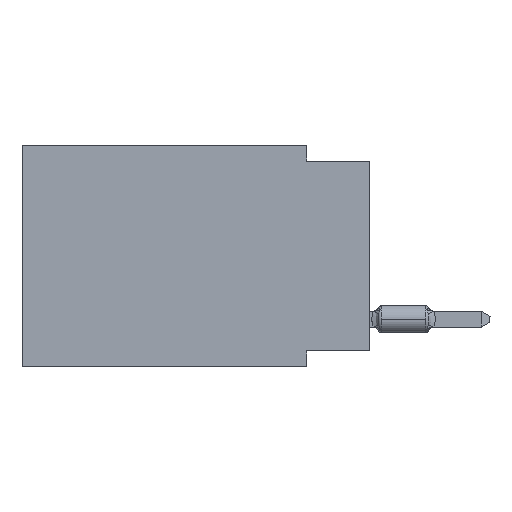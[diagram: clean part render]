
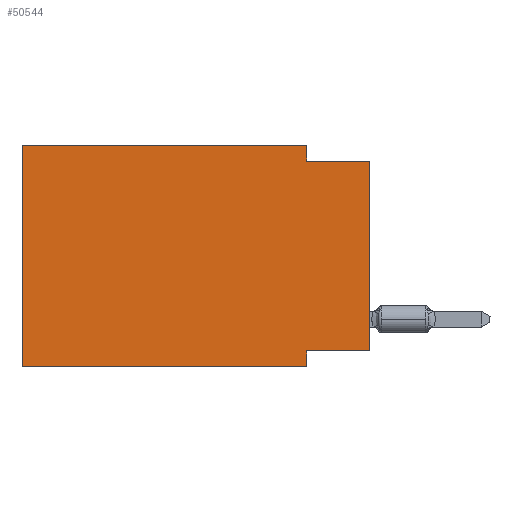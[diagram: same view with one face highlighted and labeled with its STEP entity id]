
A CAD part, left-side view. The second image highlights one B-rep face of the part: STEP entity #50544.
In plain terms, the highlighted planar face has unit normal (-1, 0, 0).
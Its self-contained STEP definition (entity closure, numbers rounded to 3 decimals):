
#319 = VECTOR ( 'NONE', #43218, 1000. ) ;
#4841 = EDGE_CURVE ( 'NONE', #57369, #77281, #84560, .T. ) ;
#5226 = EDGE_CURVE ( 'NONE', #74141, #13665, #69751, .T. ) ;
#5270 = CARTESIAN_POINT ( 'NONE',  ( 0., 0., -8.255 ) ) ;
#10536 = LINE ( 'NONE', #33897, #319 ) ;
#12109 = LINE ( 'NONE', #74909, #73997 ) ;
#13665 = VERTEX_POINT ( 'NONE', #39696 ) ;
#14472 = CARTESIAN_POINT ( 'NONE',  ( 0., 13.97, 0. ) ) ;
#18237 = DIRECTION ( 'NONE',  ( 0., -1., 0. ) ) ;
#18654 = EDGE_CURVE ( 'NONE', #75126, #88670, #10536, .T. ) ;
#21568 = EDGE_LOOP ( 'NONE', ( #23411, #101276, #94183, #102520, #75475, #31586, #55959, #97567 ) ) ;
#23411 = ORIENTED_EDGE ( 'NONE', *, *, #63049, .T. ) ;
#25244 = PLANE ( 'NONE',  #90442 ) ;
#25369 = VECTOR ( 'NONE', #18237, 1000. ) ;
#26015 = VECTOR ( 'NONE', #51516, 1000. ) ;
#31586 = ORIENTED_EDGE ( 'NONE', *, *, #64441, .T. ) ;
#33897 = CARTESIAN_POINT ( 'NONE',  ( 0., 2.54, -8.89 ) ) ;
#34335 = LINE ( 'NONE', #57688, #25369 ) ;
#34514 = DIRECTION ( 'NONE',  ( 0., 1., 0. ) ) ;
#36077 = CARTESIAN_POINT ( 'NONE',  ( 0., 2.54, -8.89 ) ) ;
#37963 = VERTEX_POINT ( 'NONE', #46831 ) ;
#39696 = CARTESIAN_POINT ( 'NONE',  ( 0., 0., -0.635 ) ) ;
#40943 = CARTESIAN_POINT ( 'NONE',  ( 0., 2.54, 0. ) ) ;
#43218 = DIRECTION ( 'NONE',  ( 0., 0., -1. ) ) ;
#43226 = CARTESIAN_POINT ( 'NONE',  ( 0., 0., 0. ) ) ;
#46831 = CARTESIAN_POINT ( 'NONE',  ( 0., 0., -8.255 ) ) ;
#47972 = EDGE_CURVE ( 'NONE', #77281, #57215, #34335, .T. ) ;
#50544 = ADVANCED_FACE ( 'NONE', ( #65697 ), #25244, .F. ) ;
#51516 = DIRECTION ( 'NONE',  ( 0., 0., 1. ) ) ;
#55959 = ORIENTED_EDGE ( 'NONE', *, *, #18654, .F. ) ;
#57215 = VERTEX_POINT ( 'NONE', #78774 ) ;
#57369 = VERTEX_POINT ( 'NONE', #77749 ) ;
#57688 = CARTESIAN_POINT ( 'NONE',  ( 0., 13.97, 0. ) ) ;
#57933 = DIRECTION ( 'NONE',  ( 0., 0., -1. ) ) ;
#63049 = EDGE_CURVE ( 'NONE', #37963, #13665, #67582, .T. ) ;
#64441 = EDGE_CURVE ( 'NONE', #57369, #88670, #12109, .T. ) ;
#64946 = VECTOR ( 'NONE', #34514, 1000. ) ;
#65697 = FACE_OUTER_BOUND ( 'NONE', #21568, .T. ) ;
#66331 = LINE ( 'NONE', #40943, #99849 ) ;
#66732 = CARTESIAN_POINT ( 'NONE',  ( 0., 13.97, 0. ) ) ;
#67582 = LINE ( 'NONE', #43226, #26015 ) ;
#69309 = CARTESIAN_POINT ( 'NONE',  ( 0., 13.97, 0. ) ) ;
#69751 = LINE ( 'NONE', #78060, #100337 ) ;
#73997 = VECTOR ( 'NONE', #82205, 1000. ) ;
#74141 = VERTEX_POINT ( 'NONE', #76071 ) ;
#74909 = CARTESIAN_POINT ( 'NONE',  ( 0., 13.97, -8.89 ) ) ;
#75126 = VERTEX_POINT ( 'NONE', #96522 ) ;
#75475 = ORIENTED_EDGE ( 'NONE', *, *, #4841, .F. ) ;
#76071 = CARTESIAN_POINT ( 'NONE',  ( 0., 2.54, -0.635 ) ) ;
#77281 = VERTEX_POINT ( 'NONE', #69309 ) ;
#77749 = CARTESIAN_POINT ( 'NONE',  ( 0., 13.97, -8.89 ) ) ;
#77886 = LINE ( 'NONE', #5270, #64946 ) ;
#78060 = CARTESIAN_POINT ( 'NONE',  ( 0., 0., -0.635 ) ) ;
#78774 = CARTESIAN_POINT ( 'NONE',  ( 0., 2.54, 0. ) ) ;
#78849 = VECTOR ( 'NONE', #92340, 1000. ) ;
#82205 = DIRECTION ( 'NONE',  ( 0., -1., 0. ) ) ;
#84560 = LINE ( 'NONE', #14472, #78849 ) ;
#88189 = DIRECTION ( 'NONE',  ( 0., 0., -1. ) ) ;
#88670 = VERTEX_POINT ( 'NONE', #36077 ) ;
#90442 = AXIS2_PLACEMENT_3D ( 'NONE', #66732, #98408, #57933 ) ;
#91047 = EDGE_CURVE ( 'NONE', #57215, #74141, #66331, .T. ) ;
#92340 = DIRECTION ( 'NONE',  ( 0., 0., 1. ) ) ;
#94183 = ORIENTED_EDGE ( 'NONE', *, *, #91047, .F. ) ;
#96522 = CARTESIAN_POINT ( 'NONE',  ( 0., 2.54, -8.255 ) ) ;
#97567 = ORIENTED_EDGE ( 'NONE', *, *, #100673, .F. ) ;
#98408 = DIRECTION ( 'NONE',  ( 1., 0., 0. ) ) ;
#99849 = VECTOR ( 'NONE', #88189, 1000. ) ;
#100337 = VECTOR ( 'NONE', #101430, 1000. ) ;
#100673 = EDGE_CURVE ( 'NONE', #37963, #75126, #77886, .T. ) ;
#101276 = ORIENTED_EDGE ( 'NONE', *, *, #5226, .F. ) ;
#101430 = DIRECTION ( 'NONE',  ( 0., -1., 0. ) ) ;
#102520 = ORIENTED_EDGE ( 'NONE', *, *, #47972, .F. ) ;
